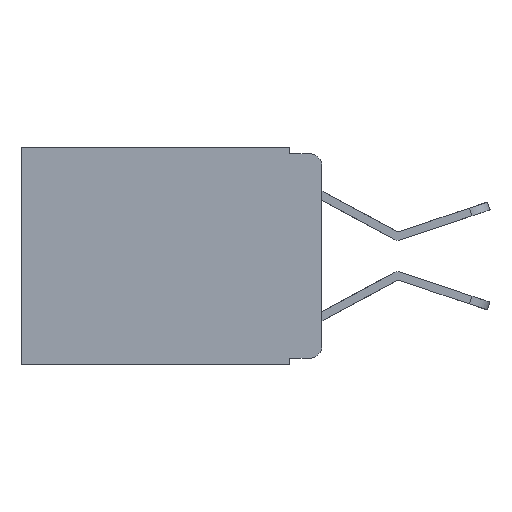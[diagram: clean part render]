
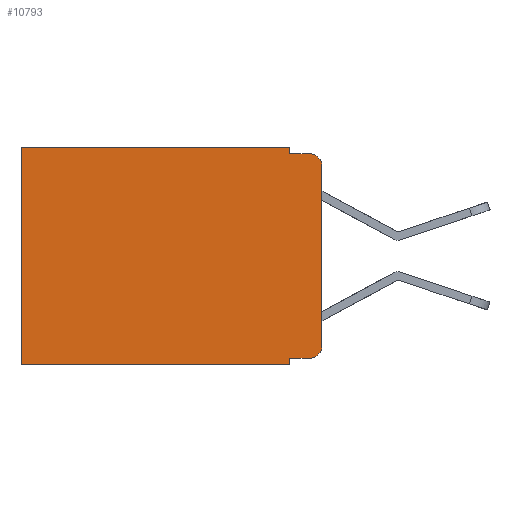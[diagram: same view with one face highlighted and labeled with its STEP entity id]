
A CAD part, left-side view. The second image highlights one B-rep face of the part: STEP entity #10793.
In plain terms, the highlighted planar face has unit normal (-1, 0, 0).
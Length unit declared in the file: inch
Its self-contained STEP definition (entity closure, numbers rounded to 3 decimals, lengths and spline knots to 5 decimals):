
#29 = VERTEX_POINT ( 'NONE', #2450 ) ;
#785 = EDGE_CURVE ( 'NONE', #29, #2266, #19791, .T. ) ;
#1073 = VECTOR ( 'NONE', #19529, 39.37008 ) ;
#1181 = VERTEX_POINT ( 'NONE', #16833 ) ;
#1320 = EDGE_CURVE ( 'NONE', #11407, #2266, #9610, .T. ) ;
#2266 = VERTEX_POINT ( 'NONE', #2284 ) ;
#2284 = CARTESIAN_POINT ( 'NONE',  ( 0.298, 0.02, -0.01 ) ) ;
#2289 = EDGE_CURVE ( 'NONE', #7545, #11702, #5056, .T. ) ;
#2450 = CARTESIAN_POINT ( 'NONE',  ( 0.298, 0., -0.03 ) ) ;
#2679 = ORIENTED_EDGE ( 'NONE', *, *, #19313, .T. ) ;
#2856 = CARTESIAN_POINT ( 'NONE',  ( 0.298, 0.02, -0.03 ) ) ;
#3096 = VECTOR ( 'NONE', #6282, 39.37008 ) ;
#3526 = LINE ( 'NONE', #14561, #8639 ) ;
#4124 = EDGE_CURVE ( 'NONE', #11273, #4941, #21691, .T. ) ;
#4459 = DIRECTION ( 'NONE',  ( 0., 1., 0. ) ) ;
#4519 = VECTOR ( 'NONE', #5095, 39.37008 ) ;
#4847 = DIRECTION ( 'NONE',  ( -1., 0., 0. ) ) ;
#4854 = ORIENTED_EDGE ( 'NONE', *, *, #8005, .F. ) ;
#4890 = CARTESIAN_POINT ( 'NONE',  ( 0.298, 0.051, 0. ) ) ;
#4941 = VERTEX_POINT ( 'NONE', #16886 ) ;
#4973 = DIRECTION ( 'NONE',  ( 0., 0., -1. ) ) ;
#5056 = LINE ( 'NONE', #6596, #4519 ) ;
#5095 = DIRECTION ( 'NONE',  ( 0., 1., 0. ) ) ;
#5459 = AXIS2_PLACEMENT_3D ( 'NONE', #15710, #5662, #17399 ) ;
#5580 = PLANE ( 'NONE',  #5459 ) ;
#5662 = DIRECTION ( 'NONE',  ( 1., 0., 0. ) ) ;
#5784 = FACE_OUTER_BOUND ( 'NONE', #14564, .T. ) ;
#6150 = EDGE_CURVE ( 'NONE', #29, #1181, #10216, .T. ) ;
#6282 = DIRECTION ( 'NONE',  ( 0., 0., -1. ) ) ;
#6465 = AXIS2_PLACEMENT_3D ( 'NONE', #8789, #20446, #10447 ) ;
#6596 = CARTESIAN_POINT ( 'NONE',  ( 0.298, 0., 0. ) ) ;
#7241 = ORIENTED_EDGE ( 'NONE', *, *, #1320, .F. ) ;
#7389 = AXIS2_PLACEMENT_3D ( 'NONE', #2856, #4847, #4973 ) ;
#7545 = VERTEX_POINT ( 'NONE', #10381 ) ;
#8005 = EDGE_CURVE ( 'NONE', #11273, #19340, #19560, .T. ) ;
#8251 = DIRECTION ( 'NONE',  ( 0., 0., -1. ) ) ;
#8333 = CARTESIAN_POINT ( 'NONE',  ( 0.298, 0.051, 0. ) ) ;
#8639 = VECTOR ( 'NONE', #4459, 39.37008 ) ;
#8789 = CARTESIAN_POINT ( 'NONE',  ( 0.298, 0.02, -0.313 ) ) ;
#8808 = ORIENTED_EDGE ( 'NONE', *, *, #19775, .F. ) ;
#8974 = VECTOR ( 'NONE', #18280, 39.37008 ) ;
#9099 = VECTOR ( 'NONE', #9999, 39.37008 ) ;
#9610 = LINE ( 'NONE', #21198, #17982 ) ;
#9999 = DIRECTION ( 'NONE',  ( 0., 0., -1. ) ) ;
#10216 = LINE ( 'NONE', #19500, #1073 ) ;
#10381 = CARTESIAN_POINT ( 'NONE',  ( 0.298, 0.051, 0. ) ) ;
#10412 = CARTESIAN_POINT ( 'NONE',  ( 0.298, 0.473, -0.343 ) ) ;
#10447 = DIRECTION ( 'NONE',  ( 0., 0., -1. ) ) ;
#10793 = ADVANCED_FACE ( 'NONE', ( #5784 ), #5580, .F. ) ;
#11273 = VERTEX_POINT ( 'NONE', #15250 ) ;
#11407 = VERTEX_POINT ( 'NONE', #15904 ) ;
#11506 = VECTOR ( 'NONE', #8251, 39.37008 ) ;
#11702 = VERTEX_POINT ( 'NONE', #16777 ) ;
#12061 = CIRCLE ( 'NONE', #6465, 0.02 ) ;
#12189 = EDGE_CURVE ( 'NONE', #11702, #17700, #16578, .T. ) ;
#13024 = ORIENTED_EDGE ( 'NONE', *, *, #14331, .F. ) ;
#14331 = EDGE_CURVE ( 'NONE', #19340, #17700, #3526, .T. ) ;
#14561 = CARTESIAN_POINT ( 'NONE',  ( 0.298, 0., -0.343 ) ) ;
#14564 = EDGE_LOOP ( 'NONE', ( #18999, #20775, #7241, #8808, #18756, #21885, #13024, #4854, #19038, #2679 ) ) ;
#14645 = CARTESIAN_POINT ( 'NONE',  ( 0.298, 0.473, 0. ) ) ;
#15250 = CARTESIAN_POINT ( 'NONE',  ( 0.298, 0.051, -0.333 ) ) ;
#15490 = CARTESIAN_POINT ( 'NONE',  ( 0.298, 0.051, -0.333 ) ) ;
#15501 = CARTESIAN_POINT ( 'NONE',  ( 0.298, 0.051, -0.343 ) ) ;
#15710 = CARTESIAN_POINT ( 'NONE',  ( 0.298, 0., 0. ) ) ;
#15904 = CARTESIAN_POINT ( 'NONE',  ( 0.298, 0.051, -0.01 ) ) ;
#15971 = LINE ( 'NONE', #4890, #11506 ) ;
#16578 = LINE ( 'NONE', #14645, #3096 ) ;
#16582 = DIRECTION ( 'NONE',  ( 0., -1., 0. ) ) ;
#16777 = CARTESIAN_POINT ( 'NONE',  ( 0.298, 0.473, 0. ) ) ;
#16833 = CARTESIAN_POINT ( 'NONE',  ( 0.298, 0., -0.313 ) ) ;
#16886 = CARTESIAN_POINT ( 'NONE',  ( 0.298, 0.02, -0.333 ) ) ;
#17399 = DIRECTION ( 'NONE',  ( 0., 0., -1. ) ) ;
#17700 = VERTEX_POINT ( 'NONE', #10412 ) ;
#17982 = VECTOR ( 'NONE', #16582, 39.37008 ) ;
#18280 = DIRECTION ( 'NONE',  ( 0., -1., 0. ) ) ;
#18756 = ORIENTED_EDGE ( 'NONE', *, *, #2289, .T. ) ;
#18999 = ORIENTED_EDGE ( 'NONE', *, *, #6150, .F. ) ;
#19038 = ORIENTED_EDGE ( 'NONE', *, *, #4124, .T. ) ;
#19313 = EDGE_CURVE ( 'NONE', #4941, #1181, #12061, .T. ) ;
#19340 = VERTEX_POINT ( 'NONE', #15501 ) ;
#19500 = CARTESIAN_POINT ( 'NONE',  ( 0.298, 0., 0. ) ) ;
#19529 = DIRECTION ( 'NONE',  ( 0., 0., -1. ) ) ;
#19560 = LINE ( 'NONE', #8333, #9099 ) ;
#19775 = EDGE_CURVE ( 'NONE', #7545, #11407, #15971, .T. ) ;
#19791 = CIRCLE ( 'NONE', #7389, 0.02 ) ;
#20446 = DIRECTION ( 'NONE',  ( -1., 0., 0. ) ) ;
#20775 = ORIENTED_EDGE ( 'NONE', *, *, #785, .T. ) ;
#21198 = CARTESIAN_POINT ( 'NONE',  ( 0.298, 0.051, -0.01 ) ) ;
#21691 = LINE ( 'NONE', #15490, #8974 ) ;
#21885 = ORIENTED_EDGE ( 'NONE', *, *, #12189, .T. ) ;
